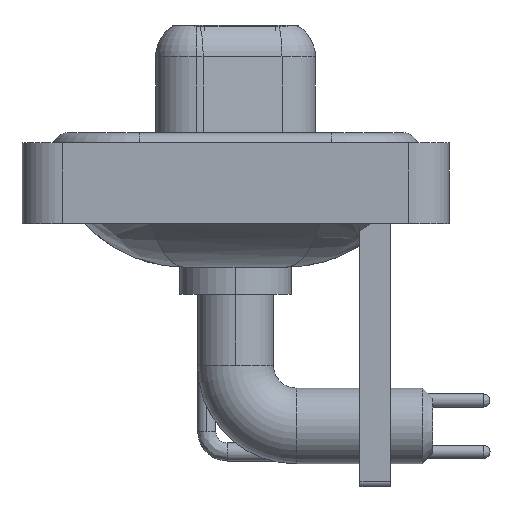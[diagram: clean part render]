
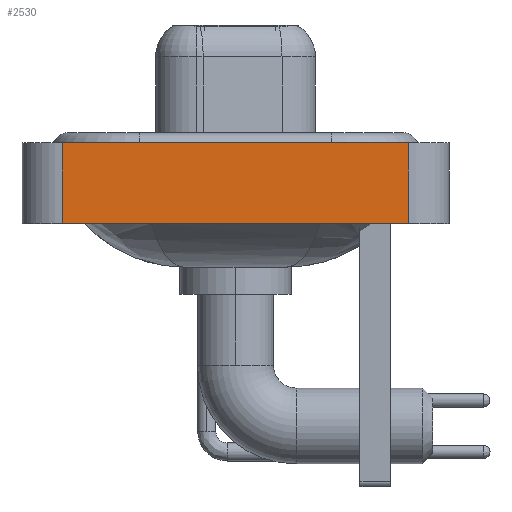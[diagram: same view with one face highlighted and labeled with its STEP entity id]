
A CAD part, left-side view. The second image highlights one B-rep face of the part: STEP entity #2530.
In plain terms, the highlighted planar face has unit normal (-1, 0, 0).
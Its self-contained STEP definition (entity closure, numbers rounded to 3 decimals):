
#1064 = LINE ( 'NONE', #14803, #6159 ) ;
#1711 = CARTESIAN_POINT ( 'NONE',  ( -7.35, -8.55, 0.4 ) ) ;
#1831 = LINE ( 'NONE', #1711, #13800 ) ;
#1925 = DIRECTION ( 'NONE',  ( 0., 0., 1. ) ) ;
#2055 = DIRECTION ( 'NONE',  ( -1., 0., 0. ) ) ;
#2530 = ADVANCED_FACE ( 'NONE', ( #16948 ), #24796, .T. ) ;
#3705 = LINE ( 'NONE', #22989, #16793 ) ;
#5182 = EDGE_LOOP ( 'NONE', ( #19309, #7737, #17688, #18665 ) ) ;
#6159 = VECTOR ( 'NONE', #6857, 1000. ) ;
#6827 = CARTESIAN_POINT ( 'NONE',  ( -7.35, 8.55, 0.4 ) ) ;
#6857 = DIRECTION ( 'NONE',  ( 0., 0., 1. ) ) ;
#7737 = ORIENTED_EDGE ( 'NONE', *, *, #11466, .F. ) ;
#8623 = VERTEX_POINT ( 'NONE', #14342 ) ;
#10043 = CARTESIAN_POINT ( 'NONE',  ( -7.35, -8.55, -3.6 ) ) ;
#10357 = AXIS2_PLACEMENT_3D ( 'NONE', #21193, #2055, #1925 ) ;
#10987 = VECTOR ( 'NONE', #15608, 1000. ) ;
#11466 = EDGE_CURVE ( 'NONE', #18753, #13811, #1831, .T. ) ;
#13645 = LINE ( 'NONE', #10043, #10987 ) ;
#13800 = VECTOR ( 'NONE', #25362, 1000. ) ;
#13811 = VERTEX_POINT ( 'NONE', #20211 ) ;
#14049 = VERTEX_POINT ( 'NONE', #19730 ) ;
#14342 = CARTESIAN_POINT ( 'NONE',  ( -7.35, -8.55, -3.6 ) ) ;
#14803 = CARTESIAN_POINT ( 'NONE',  ( -7.35, -8.55, -3.6 ) ) ;
#15608 = DIRECTION ( 'NONE',  ( 0., -1., 0. ) ) ;
#16793 = VECTOR ( 'NONE', #24915, 1000. ) ;
#16948 = FACE_OUTER_BOUND ( 'NONE', #5182, .T. ) ;
#17573 = EDGE_CURVE ( 'NONE', #8623, #13811, #1064, .T. ) ;
#17688 = ORIENTED_EDGE ( 'NONE', *, *, #21974, .F. ) ;
#18665 = ORIENTED_EDGE ( 'NONE', *, *, #20517, .T. ) ;
#18753 = VERTEX_POINT ( 'NONE', #6827 ) ;
#19309 = ORIENTED_EDGE ( 'NONE', *, *, #17573, .T. ) ;
#19730 = CARTESIAN_POINT ( 'NONE',  ( -7.35, 8.55, -3.6 ) ) ;
#20211 = CARTESIAN_POINT ( 'NONE',  ( -7.35, -8.55, 0.4 ) ) ;
#20517 = EDGE_CURVE ( 'NONE', #14049, #8623, #13645, .T. ) ;
#21193 = CARTESIAN_POINT ( 'NONE',  ( -7.35, -8.55, -3.6 ) ) ;
#21974 = EDGE_CURVE ( 'NONE', #14049, #18753, #3705, .T. ) ;
#22989 = CARTESIAN_POINT ( 'NONE',  ( -7.35, 8.55, -3.6 ) ) ;
#24796 = PLANE ( 'NONE',  #10357 ) ;
#24915 = DIRECTION ( 'NONE',  ( 0., 0., 1. ) ) ;
#25362 = DIRECTION ( 'NONE',  ( 0., -1., 0. ) ) ;
